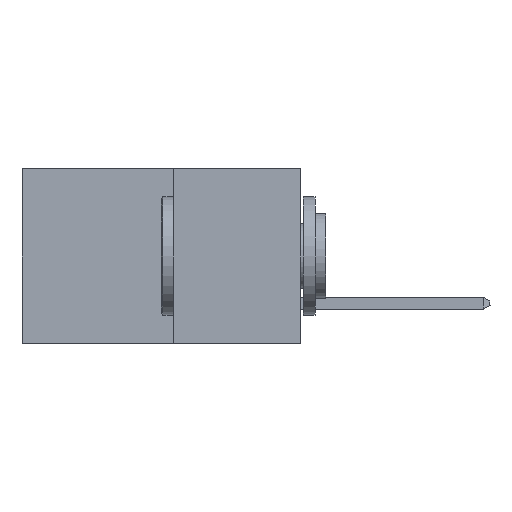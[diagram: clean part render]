
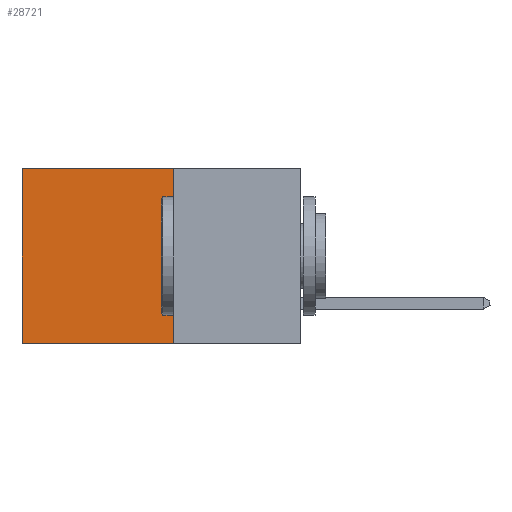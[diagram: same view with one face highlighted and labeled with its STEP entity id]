
A CAD part, left-side view. The second image highlights one B-rep face of the part: STEP entity #28721.
In plain terms, the highlighted planar face has unit normal (-1, 0, 0).
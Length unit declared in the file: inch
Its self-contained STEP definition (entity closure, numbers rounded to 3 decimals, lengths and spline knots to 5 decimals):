
#1391 = DIRECTION ( 'NONE',  ( 0., 0., -1. ) ) ;
#1486 = CARTESIAN_POINT ( 'NONE',  ( 0.277, 0.59, 0. ) ) ;
#1930 = LINE ( 'NONE', #30230, #7930 ) ;
#2834 = CARTESIAN_POINT ( 'NONE',  ( 0.277, 0.59, -0.37 ) ) ;
#3202 = EDGE_CURVE ( 'NONE', #24279, #15167, #24891, .T. ) ;
#4302 = VECTOR ( 'NONE', #14239, 39.37008 ) ;
#5871 = ORIENTED_EDGE ( 'NONE', *, *, #15900, .F. ) ;
#7930 = VECTOR ( 'NONE', #25467, 39.37008 ) ;
#8044 = CARTESIAN_POINT ( 'NONE',  ( 0.277, 0.27, -0.37 ) ) ;
#9185 = EDGE_CURVE ( 'NONE', #21921, #10112, #1930, .T. ) ;
#9247 = CARTESIAN_POINT ( 'NONE',  ( 0.277, 0.27, -0.37 ) ) ;
#9844 = DIRECTION ( 'NONE',  ( 0., 1., 0. ) ) ;
#9859 = ORIENTED_EDGE ( 'NONE', *, *, #14946, .T. ) ;
#10112 = VERTEX_POINT ( 'NONE', #2834 ) ;
#10277 = LINE ( 'NONE', #9247, #4302 ) ;
#10886 = ORIENTED_EDGE ( 'NONE', *, *, #9185, .T. ) ;
#13996 = CARTESIAN_POINT ( 'NONE',  ( 0.277, 0.27, -0.37 ) ) ;
#14239 = DIRECTION ( 'NONE',  ( 0., 1., 0. ) ) ;
#14563 = VECTOR ( 'NONE', #9844, 39.37008 ) ;
#14946 = EDGE_CURVE ( 'NONE', #24279, #21921, #27931, .T. ) ;
#15167 = VERTEX_POINT ( 'NONE', #8044 ) ;
#15900 = EDGE_CURVE ( 'NONE', #15167, #10112, #10277, .T. ) ;
#16150 = FACE_OUTER_BOUND ( 'NONE', #20570, .T. ) ;
#16483 = DIRECTION ( 'NONE',  ( 1., 0., 0. ) ) ;
#17227 = CARTESIAN_POINT ( 'NONE',  ( 0.277, 0.27, 0. ) ) ;
#18102 = VECTOR ( 'NONE', #23495, 39.37008 ) ;
#20570 = EDGE_LOOP ( 'NONE', ( #10886, #5871, #22247, #9859 ) ) ;
#21921 = VERTEX_POINT ( 'NONE', #1486 ) ;
#22247 = ORIENTED_EDGE ( 'NONE', *, *, #3202, .F. ) ;
#23495 = DIRECTION ( 'NONE',  ( 0., 0., -1. ) ) ;
#23797 = CARTESIAN_POINT ( 'NONE',  ( 0.277, 0.27, -0.37 ) ) ;
#24259 = AXIS2_PLACEMENT_3D ( 'NONE', #13996, #16483, #1391 ) ;
#24279 = VERTEX_POINT ( 'NONE', #25982 ) ;
#24891 = LINE ( 'NONE', #23797, #18102 ) ;
#25467 = DIRECTION ( 'NONE',  ( 0., 0., -1. ) ) ;
#25982 = CARTESIAN_POINT ( 'NONE',  ( 0.277, 0.27, 0. ) ) ;
#27931 = LINE ( 'NONE', #17227, #14563 ) ;
#28721 = ADVANCED_FACE ( 'NONE', ( #16150 ), #31432, .F. ) ;
#30230 = CARTESIAN_POINT ( 'NONE',  ( 0.277, 0.59, -0.37 ) ) ;
#31432 = PLANE ( 'NONE',  #24259 ) ;
